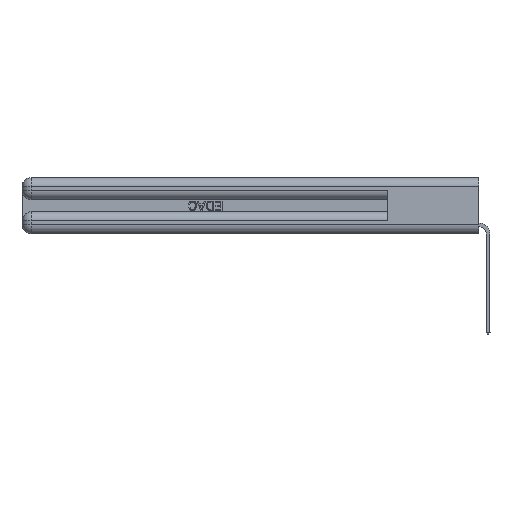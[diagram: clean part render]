
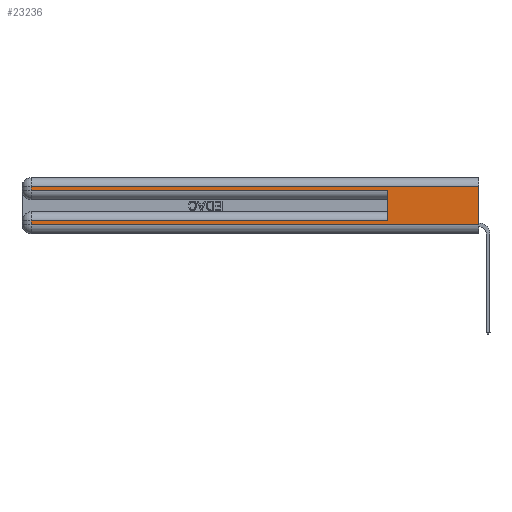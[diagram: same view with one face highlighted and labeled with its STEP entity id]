
A CAD part, left-side view. The second image highlights one B-rep face of the part: STEP entity #23236.
In plain terms, the highlighted planar face has unit normal (-1, 0, 0).
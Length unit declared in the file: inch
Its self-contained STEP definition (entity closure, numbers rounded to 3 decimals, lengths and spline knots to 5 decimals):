
#1047 = ORIENTED_EDGE ( 'NONE', *, *, #13440, .T. ) ;
#1118 = VECTOR ( 'NONE', #17794, 39.37008 ) ;
#1651 = DIRECTION ( 'NONE',  ( 0., 0., -1. ) ) ;
#1974 = VERTEX_POINT ( 'NONE', #13814 ) ;
#2198 = VERTEX_POINT ( 'NONE', #7987 ) ;
#2442 = ORIENTED_EDGE ( 'NONE', *, *, #20957, .T. ) ;
#3048 = CARTESIAN_POINT ( 'NONE',  ( 0., 0., 0.37 ) ) ;
#3171 = EDGE_LOOP ( 'NONE', ( #28884, #10124, #4281, #1047, #28666, #2442, #21274, #6690 ) ) ;
#3357 = VERTEX_POINT ( 'NONE', #27586 ) ;
#4211 = LINE ( 'NONE', #10066, #15371 ) ;
#4281 = ORIENTED_EDGE ( 'NONE', *, *, #14917, .T. ) ;
#4413 = CARTESIAN_POINT ( 'NONE',  ( 0., 0., 0.085 ) ) ;
#5183 = CARTESIAN_POINT ( 'NONE',  ( 0., 0., 0.06 ) ) ;
#5803 = CARTESIAN_POINT ( 'NONE',  ( 0., 0., 0.31 ) ) ;
#6088 = LINE ( 'NONE', #5803, #28394 ) ;
#6690 = ORIENTED_EDGE ( 'NONE', *, *, #25458, .T. ) ;
#6780 = VERTEX_POINT ( 'NONE', #23442 ) ;
#6948 = DIRECTION ( 'NONE',  ( 0., 0., -1. ) ) ;
#7119 = LINE ( 'NONE', #24456, #1118 ) ;
#7987 = CARTESIAN_POINT ( 'NONE',  ( 0., 0., 0.31 ) ) ;
#9206 = CARTESIAN_POINT ( 'NONE',  ( 0., 2.94, 0.37 ) ) ;
#10066 = CARTESIAN_POINT ( 'NONE',  ( 0., 0.6, 0.145 ) ) ;
#10124 = ORIENTED_EDGE ( 'NONE', *, *, #10494, .T. ) ;
#10494 = EDGE_CURVE ( 'NONE', #2198, #17994, #6088, .T. ) ;
#11720 = FACE_OUTER_BOUND ( 'NONE', #3171, .T. ) ;
#11962 = EDGE_CURVE ( 'NONE', #2198, #23558, #18900, .T. ) ;
#12035 = DIRECTION ( 'NONE',  ( 0., 0., -1. ) ) ;
#12342 = VECTOR ( 'NONE', #25308, 39.37008 ) ;
#12969 = VECTOR ( 'NONE', #1651, 39.37008 ) ;
#13440 = EDGE_CURVE ( 'NONE', #17942, #1974, #27754, .T. ) ;
#13597 = CARTESIAN_POINT ( 'NONE',  ( 0., 0., 0.285 ) ) ;
#13814 = CARTESIAN_POINT ( 'NONE',  ( 0., 0.6, 0.285 ) ) ;
#14917 = EDGE_CURVE ( 'NONE', #17994, #17942, #7119, .T. ) ;
#14929 = VECTOR ( 'NONE', #22306, 39.37008 ) ;
#15371 = VECTOR ( 'NONE', #27852, 39.37008 ) ;
#16440 = EDGE_CURVE ( 'NONE', #28185, #1974, #4211, .T. ) ;
#17037 = LINE ( 'NONE', #4413, #14929 ) ;
#17323 = CARTESIAN_POINT ( 'NONE',  ( 0., 2.94, 0.31 ) ) ;
#17652 = CARTESIAN_POINT ( 'NONE',  ( 0., 0., 0.06 ) ) ;
#17794 = DIRECTION ( 'NONE',  ( 0., 0., -1. ) ) ;
#17820 = LINE ( 'NONE', #9206, #21144 ) ;
#17942 = VERTEX_POINT ( 'NONE', #23902 ) ;
#17994 = VERTEX_POINT ( 'NONE', #17323 ) ;
#18269 = LINE ( 'NONE', #5183, #12342 ) ;
#18664 = PLANE ( 'NONE',  #27149 ) ;
#18900 = LINE ( 'NONE', #26186, #12969 ) ;
#19407 = EDGE_CURVE ( 'NONE', #3357, #6780, #17820, .T. ) ;
#20957 = EDGE_CURVE ( 'NONE', #28185, #3357, #17037, .T. ) ;
#21144 = VECTOR ( 'NONE', #6948, 39.37008 ) ;
#21274 = ORIENTED_EDGE ( 'NONE', *, *, #19407, .T. ) ;
#21463 = CARTESIAN_POINT ( 'NONE',  ( 0., 0.6, 0.085 ) ) ;
#22306 = DIRECTION ( 'NONE',  ( 0., 1., 0. ) ) ;
#23236 = ADVANCED_FACE ( 'NONE', ( #11720 ), #18664, .F. ) ;
#23442 = CARTESIAN_POINT ( 'NONE',  ( 0., 2.94, 0.06 ) ) ;
#23496 = DIRECTION ( 'NONE',  ( 0., 1., 0. ) ) ;
#23558 = VERTEX_POINT ( 'NONE', #17652 ) ;
#23902 = CARTESIAN_POINT ( 'NONE',  ( 0., 2.94, 0.285 ) ) ;
#24456 = CARTESIAN_POINT ( 'NONE',  ( 0., 2.94, 0.37 ) ) ;
#25308 = DIRECTION ( 'NONE',  ( 0., -1., 0. ) ) ;
#25439 = DIRECTION ( 'NONE',  ( 1., 0., 0. ) ) ;
#25458 = EDGE_CURVE ( 'NONE', #6780, #23558, #18269, .T. ) ;
#26186 = CARTESIAN_POINT ( 'NONE',  ( 0., 0., 0.37 ) ) ;
#26950 = DIRECTION ( 'NONE',  ( 0., -1., 0. ) ) ;
#27070 = VECTOR ( 'NONE', #26950, 39.37008 ) ;
#27149 = AXIS2_PLACEMENT_3D ( 'NONE', #3048, #25439, #12035 ) ;
#27586 = CARTESIAN_POINT ( 'NONE',  ( 0., 2.94, 0.085 ) ) ;
#27754 = LINE ( 'NONE', #13597, #27070 ) ;
#27852 = DIRECTION ( 'NONE',  ( 0., 0., 1. ) ) ;
#28185 = VERTEX_POINT ( 'NONE', #21463 ) ;
#28394 = VECTOR ( 'NONE', #23496, 39.37008 ) ;
#28666 = ORIENTED_EDGE ( 'NONE', *, *, #16440, .F. ) ;
#28884 = ORIENTED_EDGE ( 'NONE', *, *, #11962, .F. ) ;
